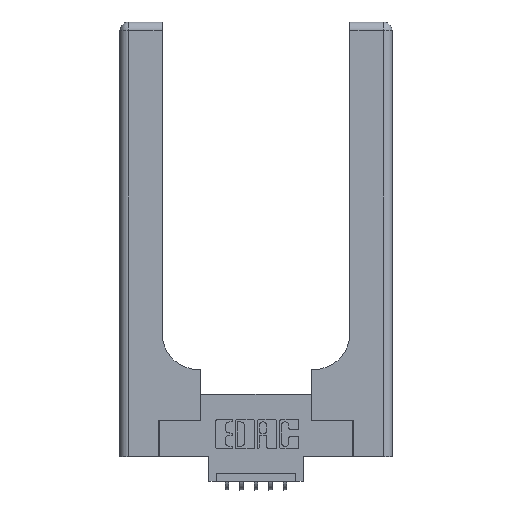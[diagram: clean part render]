
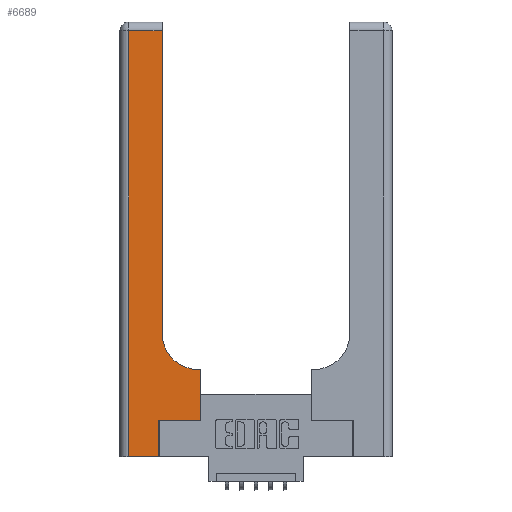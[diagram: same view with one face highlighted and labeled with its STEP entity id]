
A CAD part, top view. The second image highlights one B-rep face of the part: STEP entity #6689.
In plain terms, the highlighted planar face has unit normal (0, 0, 1).
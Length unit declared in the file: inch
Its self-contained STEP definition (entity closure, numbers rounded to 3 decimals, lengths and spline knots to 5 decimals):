
#24 = LINE ( 'NONE', #5971, #11337 ) ;
#36 = DIRECTION ( 'NONE',  ( 0., 0., -1. ) ) ;
#371 = EDGE_LOOP ( 'NONE', ( #4585, #2578, #14120, #4086, #13727, #3562, #10288, #4115, #1101 ) ) ;
#489 = DIRECTION ( 'NONE',  ( 0., 1., 0. ) ) ;
#781 = VECTOR ( 'NONE', #6618, 39.37008 ) ;
#1101 = ORIENTED_EDGE ( 'NONE', *, *, #13890, .T. ) ;
#1105 = EDGE_CURVE ( 'NONE', #10163, #13432, #2855, .T. ) ;
#1126 = EDGE_CURVE ( 'NONE', #12303, #11772, #1662, .T. ) ;
#1542 = CARTESIAN_POINT ( 'NONE',  ( 0.2915, 3., 0.37 ) ) ;
#1662 = LINE ( 'NONE', #10494, #3702 ) ;
#1801 = CARTESIAN_POINT ( 'NONE',  ( 0.269, 0., 0.37 ) ) ;
#2175 = CARTESIAN_POINT ( 'NONE',  ( 0., 2.94, 0.37 ) ) ;
#2578 = ORIENTED_EDGE ( 'NONE', *, *, #5464, .T. ) ;
#2711 = CARTESIAN_POINT ( 'NONE',  ( 0.5415, 0.6, 0.37 ) ) ;
#2792 = VECTOR ( 'NONE', #12462, 39.37008 ) ;
#2855 = LINE ( 'NONE', #1542, #4551 ) ;
#3312 = VERTEX_POINT ( 'NONE', #4280 ) ;
#3456 = VERTEX_POINT ( 'NONE', #2711 ) ;
#3562 = ORIENTED_EDGE ( 'NONE', *, *, #12253, .T. ) ;
#3663 = CARTESIAN_POINT ( 'NONE',  ( 0.06, 3., 0.37 ) ) ;
#3702 = VECTOR ( 'NONE', #6116, 39.37008 ) ;
#4016 = CARTESIAN_POINT ( 'NONE',  ( 0.269, 0.25, 0.37 ) ) ;
#4086 = ORIENTED_EDGE ( 'NONE', *, *, #4119, .T. ) ;
#4115 = ORIENTED_EDGE ( 'NONE', *, *, #7559, .T. ) ;
#4119 = EDGE_CURVE ( 'NONE', #11027, #3312, #24, .T. ) ;
#4229 = VECTOR ( 'NONE', #11785, 39.37008 ) ;
#4237 = PLANE ( 'NONE',  #8231 ) ;
#4280 = CARTESIAN_POINT ( 'NONE',  ( 0.269, 0., 0.37 ) ) ;
#4342 = LINE ( 'NONE', #13214, #781 ) ;
#4551 = VECTOR ( 'NONE', #489, 39.37008 ) ;
#4585 = ORIENTED_EDGE ( 'NONE', *, *, #1105, .T. ) ;
#5382 = CARTESIAN_POINT ( 'NONE',  ( 0., 3., 0.37 ) ) ;
#5409 = FACE_OUTER_BOUND ( 'NONE', #371, .T. ) ;
#5464 = EDGE_CURVE ( 'NONE', #13432, #9485, #8722, .T. ) ;
#5617 = AXIS2_PLACEMENT_3D ( 'NONE', #7538, #36, #12050 ) ;
#5798 = EDGE_CURVE ( 'NONE', #3312, #7971, #6638, .T. ) ;
#5971 = CARTESIAN_POINT ( 'NONE',  ( 0., 0., 0.37 ) ) ;
#6116 = DIRECTION ( 'NONE',  ( 0., 1., 0. ) ) ;
#6618 = DIRECTION ( 'NONE',  ( -1., 0., 0. ) ) ;
#6623 = LINE ( 'NONE', #4016, #7811 ) ;
#6638 = LINE ( 'NONE', #1801, #4229 ) ;
#6689 = ADVANCED_FACE ( 'NONE', ( #5409 ), #4237, .F. ) ;
#6754 = CARTESIAN_POINT ( 'NONE',  ( 0.5585, 0.6, 0.37 ) ) ;
#7147 = VECTOR ( 'NONE', #13221, 39.37008 ) ;
#7538 = CARTESIAN_POINT ( 'NONE',  ( 0.5415, 0.85, 0.37 ) ) ;
#7559 = EDGE_CURVE ( 'NONE', #11772, #3456, #4342, .T. ) ;
#7759 = CARTESIAN_POINT ( 'NONE',  ( 0.2915, 2.94, 0.37 ) ) ;
#7811 = VECTOR ( 'NONE', #11813, 39.37008 ) ;
#7901 = CARTESIAN_POINT ( 'NONE',  ( 0.2915, 0.85, 0.37 ) ) ;
#7971 = VERTEX_POINT ( 'NONE', #9007 ) ;
#8231 = AXIS2_PLACEMENT_3D ( 'NONE', #5382, #8668, #14063 ) ;
#8436 = CARTESIAN_POINT ( 'NONE',  ( 0.06, 0., 0.37 ) ) ;
#8668 = DIRECTION ( 'NONE',  ( 0., 0., -1. ) ) ;
#8718 = EDGE_CURVE ( 'NONE', #9485, #11027, #9305, .T. ) ;
#8722 = LINE ( 'NONE', #2175, #7147 ) ;
#9007 = CARTESIAN_POINT ( 'NONE',  ( 0.269, 0.25, 0.37 ) ) ;
#9292 = DIRECTION ( 'NONE',  ( 1., 0., 0. ) ) ;
#9305 = LINE ( 'NONE', #3663, #2792 ) ;
#9485 = VERTEX_POINT ( 'NONE', #10640 ) ;
#9504 = CIRCLE ( 'NONE', #5617, 0.25 ) ;
#10163 = VERTEX_POINT ( 'NONE', #7901 ) ;
#10288 = ORIENTED_EDGE ( 'NONE', *, *, #1126, .T. ) ;
#10494 = CARTESIAN_POINT ( 'NONE',  ( 0.5585, 0.25, 0.37 ) ) ;
#10640 = CARTESIAN_POINT ( 'NONE',  ( 0.06, 2.94, 0.37 ) ) ;
#11027 = VERTEX_POINT ( 'NONE', #8436 ) ;
#11337 = VECTOR ( 'NONE', #9292, 39.37008 ) ;
#11772 = VERTEX_POINT ( 'NONE', #6754 ) ;
#11785 = DIRECTION ( 'NONE',  ( 0., 1., 0. ) ) ;
#11813 = DIRECTION ( 'NONE',  ( 1., 0., 0. ) ) ;
#12047 = CARTESIAN_POINT ( 'NONE',  ( 0.5585, 0.25, 0.37 ) ) ;
#12050 = DIRECTION ( 'NONE',  ( 1., 0., 0. ) ) ;
#12253 = EDGE_CURVE ( 'NONE', #7971, #12303, #6623, .T. ) ;
#12303 = VERTEX_POINT ( 'NONE', #12047 ) ;
#12462 = DIRECTION ( 'NONE',  ( 0., -1., 0. ) ) ;
#13214 = CARTESIAN_POINT ( 'NONE',  ( 0.2915, 0.6, 0.37 ) ) ;
#13221 = DIRECTION ( 'NONE',  ( -1., 0., 0. ) ) ;
#13432 = VERTEX_POINT ( 'NONE', #7759 ) ;
#13727 = ORIENTED_EDGE ( 'NONE', *, *, #5798, .T. ) ;
#13890 = EDGE_CURVE ( 'NONE', #3456, #10163, #9504, .T. ) ;
#14063 = DIRECTION ( 'NONE',  ( -1., 0., 0. ) ) ;
#14120 = ORIENTED_EDGE ( 'NONE', *, *, #8718, .T. ) ;
